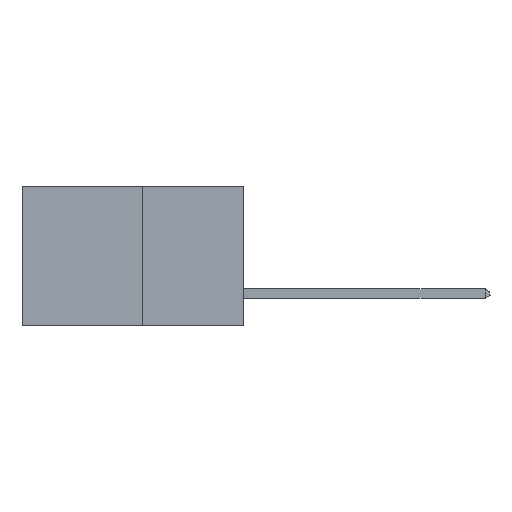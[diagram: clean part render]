
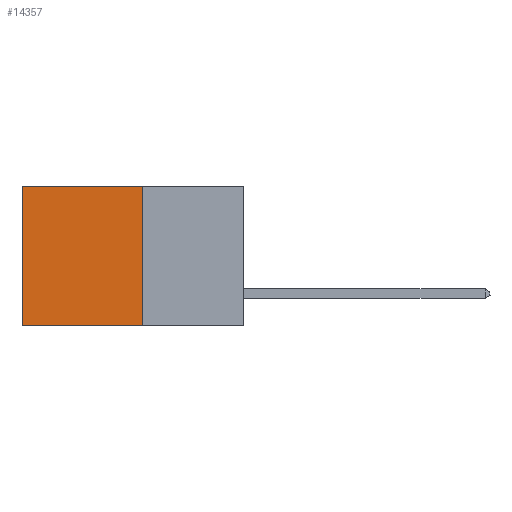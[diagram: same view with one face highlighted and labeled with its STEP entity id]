
A CAD part, left-side view. The second image highlights one B-rep face of the part: STEP entity #14357.
In plain terms, the highlighted planar face has unit normal (-1, 0, 0).
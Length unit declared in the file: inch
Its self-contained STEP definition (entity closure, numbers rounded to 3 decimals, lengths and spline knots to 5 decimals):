
#978 = VERTEX_POINT ( 'NONE', #31461 ) ;
#2791 = CARTESIAN_POINT ( 'NONE',  ( 0.277, 0.27, -0.37 ) ) ;
#2894 = LINE ( 'NONE', #16764, #23060 ) ;
#2904 = ORIENTED_EDGE ( 'NONE', *, *, #25833, .F. ) ;
#3251 = VERTEX_POINT ( 'NONE', #18240 ) ;
#3522 = EDGE_CURVE ( 'NONE', #6093, #3251, #29650, .T. ) ;
#5240 = PLANE ( 'NONE',  #15265 ) ;
#5347 = DIRECTION ( 'NONE',  ( 1., 0., 0. ) ) ;
#5368 = DIRECTION ( 'NONE',  ( 0., 0., -1. ) ) ;
#6093 = VERTEX_POINT ( 'NONE', #13346 ) ;
#7716 = CARTESIAN_POINT ( 'NONE',  ( 0.277, 0.59, -0.37 ) ) ;
#8624 = VERTEX_POINT ( 'NONE', #7716 ) ;
#8734 = CARTESIAN_POINT ( 'NONE',  ( 0.277, 0.27, -0.37 ) ) ;
#9859 = ORIENTED_EDGE ( 'NONE', *, *, #22394, .T. ) ;
#13346 = CARTESIAN_POINT ( 'NONE',  ( 0.277, 0.27, 0. ) ) ;
#14357 = ADVANCED_FACE ( 'NONE', ( #32119 ), #5240, .F. ) ;
#15265 = AXIS2_PLACEMENT_3D ( 'NONE', #18425, #5347, #23690 ) ;
#15849 = LINE ( 'NONE', #2791, #21147 ) ;
#16581 = VECTOR ( 'NONE', #19123, 39.37008 ) ;
#16764 = CARTESIAN_POINT ( 'NONE',  ( 0.277, 0.27, 0. ) ) ;
#18240 = CARTESIAN_POINT ( 'NONE',  ( 0.277, 0.27, -0.37 ) ) ;
#18425 = CARTESIAN_POINT ( 'NONE',  ( 0.277, 0.27, -0.37 ) ) ;
#18557 = DIRECTION ( 'NONE',  ( 0., 1., 0. ) ) ;
#19123 = DIRECTION ( 'NONE',  ( 0., 0., -1. ) ) ;
#19767 = VECTOR ( 'NONE', #5368, 39.37008 ) ;
#19824 = ORIENTED_EDGE ( 'NONE', *, *, #3522, .F. ) ;
#21147 = VECTOR ( 'NONE', #18557, 39.37008 ) ;
#21909 = ORIENTED_EDGE ( 'NONE', *, *, #21978, .T. ) ;
#21978 = EDGE_CURVE ( 'NONE', #6093, #978, #2894, .T. ) ;
#22394 = EDGE_CURVE ( 'NONE', #978, #8624, #27571, .T. ) ;
#22877 = EDGE_LOOP ( 'NONE', ( #9859, #2904, #19824, #21909 ) ) ;
#23060 = VECTOR ( 'NONE', #27193, 39.37008 ) ;
#23690 = DIRECTION ( 'NONE',  ( 0., 0., -1. ) ) ;
#25833 = EDGE_CURVE ( 'NONE', #3251, #8624, #15849, .T. ) ;
#26253 = CARTESIAN_POINT ( 'NONE',  ( 0.277, 0.59, -0.37 ) ) ;
#27193 = DIRECTION ( 'NONE',  ( 0., 1., 0. ) ) ;
#27571 = LINE ( 'NONE', #26253, #19767 ) ;
#29650 = LINE ( 'NONE', #8734, #16581 ) ;
#31461 = CARTESIAN_POINT ( 'NONE',  ( 0.277, 0.59, 0. ) ) ;
#32119 = FACE_OUTER_BOUND ( 'NONE', #22877, .T. ) ;
